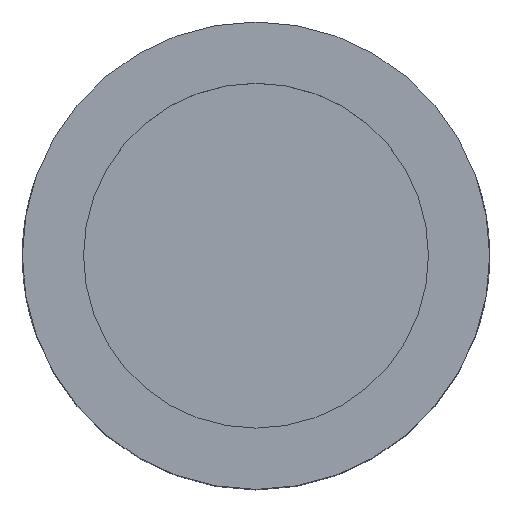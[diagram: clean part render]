
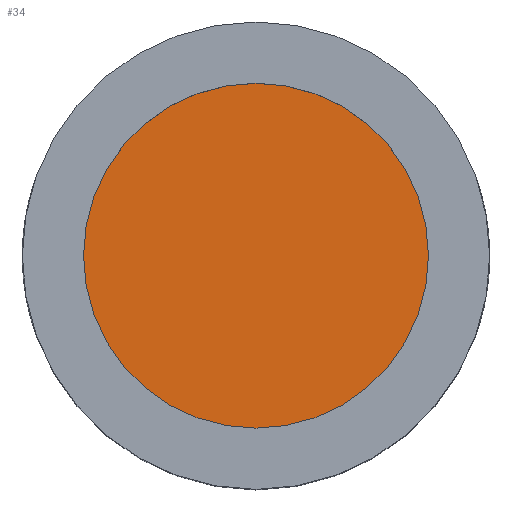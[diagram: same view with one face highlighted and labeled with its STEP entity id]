
A CAD part, top view. The second image highlights one B-rep face of the part: STEP entity #34.
In plain terms, the highlighted planar face has unit normal (0, 0, 1).
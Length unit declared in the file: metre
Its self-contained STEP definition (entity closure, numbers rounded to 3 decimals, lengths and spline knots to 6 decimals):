
#34 = ADVANCED_FACE( '', ( #68 ), #69, .T. );
#68 = FACE_OUTER_BOUND( '', #99, .T. );
#69 = PLANE( '', #100 );
#99 = EDGE_LOOP( '', ( #128 ) );
#100 = AXIS2_PLACEMENT_3D( '', #129, #130, #131 );
#128 = ORIENTED_EDGE( '', *, *, #157, .T. );
#129 = CARTESIAN_POINT( '', ( 0., 0., 0.007 ) );
#130 = DIRECTION( '', ( 0., 0., 1. ) );
#131 = DIRECTION( '', ( 1., 0., 0. ) );
#157 = EDGE_CURVE( '', #173, #173, #174, .T. );
#173 = VERTEX_POINT( '', #297 );
#174 = CIRCLE( '', #298, 0.003875 );
#297 = CARTESIAN_POINT( '', ( 0.003875, 0., 0.007 ) );
#298 = AXIS2_PLACEMENT_3D( '', #310, #311, #312 );
#310 = CARTESIAN_POINT( '', ( 0., 0., 0.007 ) );
#311 = DIRECTION( '', ( 0., 0., 1. ) );
#312 = DIRECTION( '', ( 1., 0., 0. ) );
